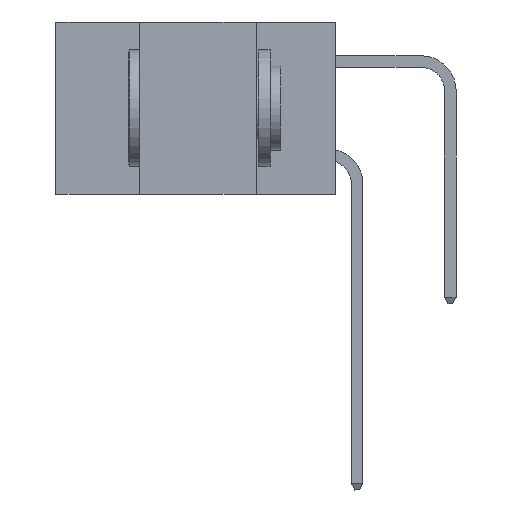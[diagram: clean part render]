
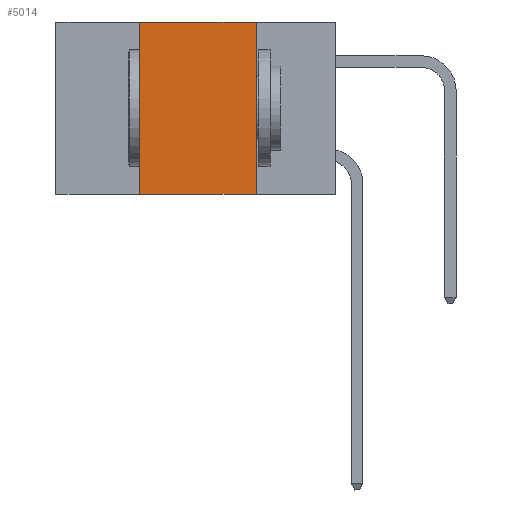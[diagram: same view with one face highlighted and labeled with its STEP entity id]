
A CAD part, left-side view. The second image highlights one B-rep face of the part: STEP entity #5014.
In plain terms, the highlighted planar face has unit normal (-1, 0, 0).
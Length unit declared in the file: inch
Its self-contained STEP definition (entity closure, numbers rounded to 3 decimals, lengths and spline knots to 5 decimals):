
#279 = DIRECTION ( 'NONE',  ( 0., -1., 0. ) ) ;
#356 = ORIENTED_EDGE ( 'NONE', *, *, #10485, .F. ) ;
#502 = CARTESIAN_POINT ( 'NONE',  ( 0., 0.17, 0. ) ) ;
#1623 = VERTEX_POINT ( 'NONE', #9677 ) ;
#1634 = AXIS2_PLACEMENT_3D ( 'NONE', #11686, #8926, #2725 ) ;
#2447 = ORIENTED_EDGE ( 'NONE', *, *, #6074, .F. ) ;
#2639 = CARTESIAN_POINT ( 'NONE',  ( 0., 0.6, 0. ) ) ;
#2725 = DIRECTION ( 'NONE',  ( 0., 0., -1. ) ) ;
#2727 = FACE_OUTER_BOUND ( 'NONE', #11458, .T. ) ;
#3869 = EDGE_CURVE ( 'NONE', #10253, #10546, #11135, .T. ) ;
#3927 = VECTOR ( 'NONE', #5548, 39.37008 ) ;
#3985 = VERTEX_POINT ( 'NONE', #10243 ) ;
#4166 = DIRECTION ( 'NONE',  ( 0., -1., 0. ) ) ;
#4908 = ORIENTED_EDGE ( 'NONE', *, *, #3869, .F. ) ;
#5014 = ADVANCED_FACE ( 'NONE', ( #2727 ), #12621, .F. ) ;
#5548 = DIRECTION ( 'NONE',  ( 0., 0., -1. ) ) ;
#5632 = CARTESIAN_POINT ( 'NONE',  ( 0., 0.17, 0. ) ) ;
#5986 = VECTOR ( 'NONE', #4166, 39.37008 ) ;
#6074 = EDGE_CURVE ( 'NONE', #1623, #10253, #10058, .T. ) ;
#6348 = EDGE_CURVE ( 'NONE', #1623, #3985, #9307, .T. ) ;
#6449 = LINE ( 'NONE', #502, #3927 ) ;
#6685 = VECTOR ( 'NONE', #279, 39.37008 ) ;
#7007 = DIRECTION ( 'NONE',  ( 0., 0., 1. ) ) ;
#8245 = CARTESIAN_POINT ( 'NONE',  ( 0., 0.42, 0. ) ) ;
#8926 = DIRECTION ( 'NONE',  ( 1., 0., 0. ) ) ;
#9307 = LINE ( 'NONE', #11109, #6685 ) ;
#9677 = CARTESIAN_POINT ( 'NONE',  ( 0., 0.42, -0.37 ) ) ;
#9887 = CARTESIAN_POINT ( 'NONE',  ( 0., 0.42, 0. ) ) ;
#10058 = LINE ( 'NONE', #9887, #11901 ) ;
#10243 = CARTESIAN_POINT ( 'NONE',  ( 0., 0.17, -0.37 ) ) ;
#10253 = VERTEX_POINT ( 'NONE', #8245 ) ;
#10485 = EDGE_CURVE ( 'NONE', #10546, #3985, #6449, .T. ) ;
#10546 = VERTEX_POINT ( 'NONE', #5632 ) ;
#11109 = CARTESIAN_POINT ( 'NONE',  ( 0., 0.6, -0.37 ) ) ;
#11135 = LINE ( 'NONE', #2639, #5986 ) ;
#11458 = EDGE_LOOP ( 'NONE', ( #356, #4908, #2447, #11747 ) ) ;
#11686 = CARTESIAN_POINT ( 'NONE',  ( 0., 0.6, 0. ) ) ;
#11747 = ORIENTED_EDGE ( 'NONE', *, *, #6348, .T. ) ;
#11901 = VECTOR ( 'NONE', #7007, 39.37008 ) ;
#12621 = PLANE ( 'NONE',  #1634 ) ;
